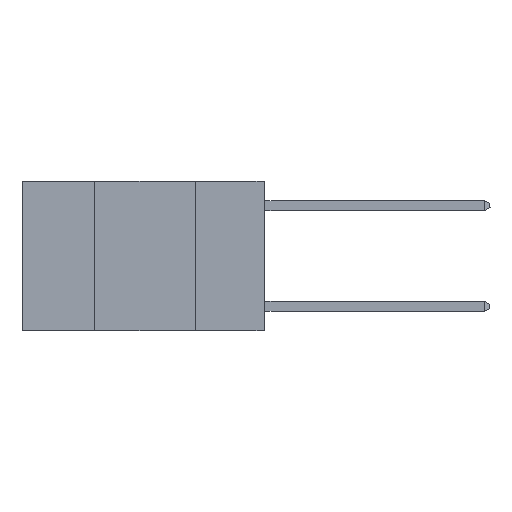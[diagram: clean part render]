
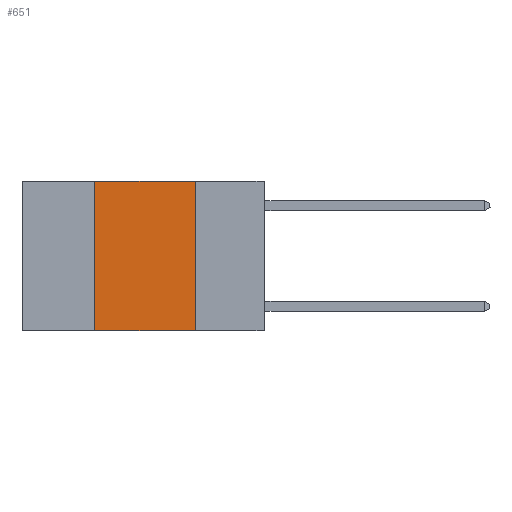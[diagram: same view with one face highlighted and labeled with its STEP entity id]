
A CAD part, left-side view. The second image highlights one B-rep face of the part: STEP entity #651.
In plain terms, the highlighted planar face has unit normal (-1, 0, 0).
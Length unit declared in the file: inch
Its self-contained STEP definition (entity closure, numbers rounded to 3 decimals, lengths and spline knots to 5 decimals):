
#105 = CARTESIAN_POINT ( 'NONE',  ( 0., 0.42, 0. ) ) ;
#651 = ADVANCED_FACE ( 'NONE', ( #7397 ), #9039, .F. ) ;
#974 = CARTESIAN_POINT ( 'NONE',  ( 0., 0.42, 0. ) ) ;
#1187 = ORIENTED_EDGE ( 'NONE', *, *, #4118, .F. ) ;
#1368 = CARTESIAN_POINT ( 'NONE',  ( 0., 0.17, -0.37 ) ) ;
#1374 = VERTEX_POINT ( 'NONE', #1368 ) ;
#1812 = CARTESIAN_POINT ( 'NONE',  ( 0., 0.6, 0. ) ) ;
#2706 = DIRECTION ( 'NONE',  ( 0., 0., 1. ) ) ;
#3431 = VECTOR ( 'NONE', #5974, 39.37008 ) ;
#3692 = EDGE_LOOP ( 'NONE', ( #5274, #1187, #8325, #6092 ) ) ;
#3982 = EDGE_CURVE ( 'NONE', #7764, #1374, #6023, .T. ) ;
#4118 = EDGE_CURVE ( 'NONE', #8016, #7764, #8935, .T. ) ;
#4777 = DIRECTION ( 'NONE',  ( 0., 0., -1. ) ) ;
#4973 = CARTESIAN_POINT ( 'NONE',  ( 0., 0.17, 0. ) ) ;
#5101 = CARTESIAN_POINT ( 'NONE',  ( 0., 0.17, 0. ) ) ;
#5274 = ORIENTED_EDGE ( 'NONE', *, *, #3982, .F. ) ;
#5746 = CARTESIAN_POINT ( 'NONE',  ( 0., 0.6, -0.37 ) ) ;
#5858 = LINE ( 'NONE', #5746, #6119 ) ;
#5974 = DIRECTION ( 'NONE',  ( 0., 0., -1. ) ) ;
#6023 = LINE ( 'NONE', #5101, #3431 ) ;
#6092 = ORIENTED_EDGE ( 'NONE', *, *, #7665, .T. ) ;
#6119 = VECTOR ( 'NONE', #8210, 39.37008 ) ;
#6398 = CARTESIAN_POINT ( 'NONE',  ( 0., 0.42, -0.37 ) ) ;
#6681 = VECTOR ( 'NONE', #6994, 39.37008 ) ;
#6974 = VERTEX_POINT ( 'NONE', #6398 ) ;
#6994 = DIRECTION ( 'NONE',  ( 0., -1., 0. ) ) ;
#7397 = FACE_OUTER_BOUND ( 'NONE', #3692, .T. ) ;
#7665 = EDGE_CURVE ( 'NONE', #6974, #1374, #5858, .T. ) ;
#7764 = VERTEX_POINT ( 'NONE', #4973 ) ;
#8016 = VERTEX_POINT ( 'NONE', #974 ) ;
#8210 = DIRECTION ( 'NONE',  ( 0., -1., 0. ) ) ;
#8325 = ORIENTED_EDGE ( 'NONE', *, *, #10421, .F. ) ;
#8918 = AXIS2_PLACEMENT_3D ( 'NONE', #10747, #9927, #4777 ) ;
#8935 = LINE ( 'NONE', #1812, #6681 ) ;
#9001 = VECTOR ( 'NONE', #2706, 39.37008 ) ;
#9039 = PLANE ( 'NONE',  #8918 ) ;
#9270 = LINE ( 'NONE', #105, #9001 ) ;
#9927 = DIRECTION ( 'NONE',  ( 1., 0., 0. ) ) ;
#10421 = EDGE_CURVE ( 'NONE', #6974, #8016, #9270, .T. ) ;
#10747 = CARTESIAN_POINT ( 'NONE',  ( 0., 0.6, 0. ) ) ;
